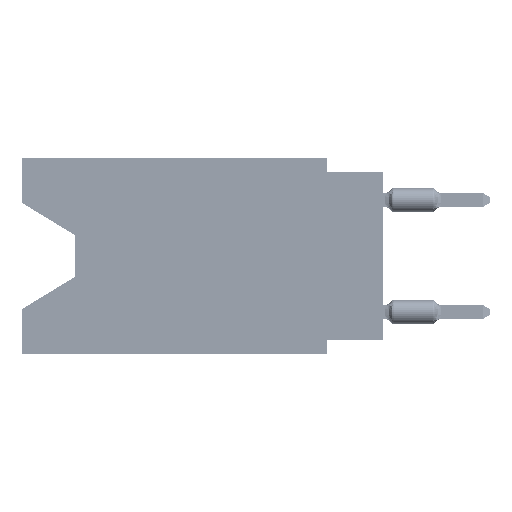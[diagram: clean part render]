
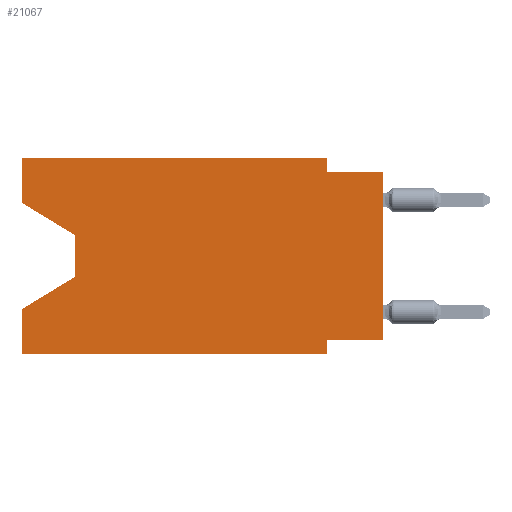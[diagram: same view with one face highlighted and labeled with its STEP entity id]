
A CAD part, left-side view. The second image highlights one B-rep face of the part: STEP entity #21067.
In plain terms, the highlighted planar face has unit normal (-1, 0, 0).
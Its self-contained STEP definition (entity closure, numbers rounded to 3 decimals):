
#1069 = DIRECTION ( 'NONE',  ( 0., -0.855, -0.519 ) ) ;
#2312 = EDGE_CURVE ( 'NONE', #9197, #61642, #28352, .T. ) ;
#5440 = DIRECTION ( 'NONE',  ( 0., 1., 0. ) ) ;
#7209 = LINE ( 'NONE', #52295, #49296 ) ;
#7264 = LINE ( 'NONE', #97376, #94020 ) ;
#8299 = VERTEX_POINT ( 'NONE', #86660 ) ;
#9197 = VERTEX_POINT ( 'NONE', #35222 ) ;
#9353 = EDGE_CURVE ( 'NONE', #62668, #56222, #99174, .T. ) ;
#10160 = VECTOR ( 'NONE', #47210, 1000. ) ;
#11792 = VECTOR ( 'NONE', #5440, 1000. ) ;
#11916 = EDGE_CURVE ( 'NONE', #56222, #8299, #92805, .T. ) ;
#14331 = CARTESIAN_POINT ( 'NONE',  ( 0., 0., -8.255 ) ) ;
#15845 = VECTOR ( 'NONE', #57086, 1000. ) ;
#16177 = DIRECTION ( 'NONE',  ( 0., 0., 1. ) ) ;
#17160 = VECTOR ( 'NONE', #99667, 1000. ) ;
#17402 = LINE ( 'NONE', #63619, #22855 ) ;
#17681 = ORIENTED_EDGE ( 'NONE', *, *, #2312, .F. ) ;
#17985 = CARTESIAN_POINT ( 'NONE',  ( 0., 13.97, -3.505 ) ) ;
#19372 = ORIENTED_EDGE ( 'NONE', *, *, #9353, .F. ) ;
#20920 = LINE ( 'NONE', #110980, #15845 ) ;
#21067 = ADVANCED_FACE ( 'NONE', ( #76289 ), #112415, .F. ) ;
#21550 = VECTOR ( 'NONE', #55060, 1000. ) ;
#22855 = VECTOR ( 'NONE', #36965, 1000. ) ;
#23311 = EDGE_CURVE ( 'NONE', #47791, #34414, #20920, .T. ) ;
#26901 = EDGE_CURVE ( 'NONE', #94471, #62668, #17402, .T. ) ;
#27769 = DIRECTION ( 'NONE',  ( 0., 0., -1. ) ) ;
#28352 = LINE ( 'NONE', #108926, #107234 ) ;
#28545 = EDGE_CURVE ( 'NONE', #50113, #61642, #7209, .T. ) ;
#32169 = LINE ( 'NONE', #14331, #11792 ) ;
#33930 = ORIENTED_EDGE ( 'NONE', *, *, #49506, .T. ) ;
#34414 = VERTEX_POINT ( 'NONE', #98135 ) ;
#35222 = CARTESIAN_POINT ( 'NONE',  ( 0., 2.54, -8.255 ) ) ;
#35524 = CARTESIAN_POINT ( 'NONE',  ( 0., 16.383, 0. ) ) ;
#36965 = DIRECTION ( 'NONE',  ( 0., -1., 0. ) ) ;
#38448 = VECTOR ( 'NONE', #73709, 1000. ) ;
#38910 = CARTESIAN_POINT ( 'NONE',  ( 0., 0., -0.635 ) ) ;
#40034 = VERTEX_POINT ( 'NONE', #108774 ) ;
#40104 = CARTESIAN_POINT ( 'NONE',  ( 0., 2.54, -8.89 ) ) ;
#45373 = CARTESIAN_POINT ( 'NONE',  ( 0., 16.383, 0. ) ) ;
#47210 = DIRECTION ( 'NONE',  ( 0., -1., 0. ) ) ;
#47679 = VERTEX_POINT ( 'NONE', #94489 ) ;
#47791 = VERTEX_POINT ( 'NONE', #17985 ) ;
#47864 = CARTESIAN_POINT ( 'NONE',  ( 0., 16.383, 0. ) ) ;
#49296 = VECTOR ( 'NONE', #88410, 1000. ) ;
#49506 = EDGE_CURVE ( 'NONE', #40034, #47791, #82264, .T. ) ;
#50113 = VERTEX_POINT ( 'NONE', #70050 ) ;
#52295 = CARTESIAN_POINT ( 'NONE',  ( 0., 16.383, -8.89 ) ) ;
#54598 = VERTEX_POINT ( 'NONE', #93763 ) ;
#55060 = DIRECTION ( 'NONE',  ( 0., 0., 1. ) ) ;
#56222 = VERTEX_POINT ( 'NONE', #82944 ) ;
#56693 = ORIENTED_EDGE ( 'NONE', *, *, #11916, .F. ) ;
#56772 = VECTOR ( 'NONE', #1069, 1000. ) ;
#57086 = DIRECTION ( 'NONE',  ( 0., 0., -1. ) ) ;
#57155 = AXIS2_PLACEMENT_3D ( 'NONE', #47864, #86310, #104099 ) ;
#57441 = LINE ( 'NONE', #103031, #89751 ) ;
#57734 = EDGE_CURVE ( 'NONE', #50113, #47679, #7264, .T. ) ;
#60188 = ORIENTED_EDGE ( 'NONE', *, *, #108642, .T. ) ;
#61642 = VERTEX_POINT ( 'NONE', #40104 ) ;
#62668 = VERTEX_POINT ( 'NONE', #64598 ) ;
#63619 = CARTESIAN_POINT ( 'NONE',  ( 0., 16.383, 0. ) ) ;
#64598 = CARTESIAN_POINT ( 'NONE',  ( 0., 2.54, 0. ) ) ;
#67486 = DIRECTION ( 'NONE',  ( 0., 0., 1. ) ) ;
#68733 = EDGE_LOOP ( 'NONE', ( #33930, #86900, #96023, #110494, #102686, #17681, #106634, #60188, #56693, #19372, #114359, #69051 ) ) ;
#69051 = ORIENTED_EDGE ( 'NONE', *, *, #92072, .F. ) ;
#70050 = CARTESIAN_POINT ( 'NONE',  ( 0., 16.383, -8.89 ) ) ;
#71059 = EDGE_CURVE ( 'NONE', #34414, #47679, #91371, .T. ) ;
#73263 = EDGE_CURVE ( 'NONE', #54598, #9197, #32169, .T. ) ;
#73709 = DIRECTION ( 'NONE',  ( 0., 0., -1. ) ) ;
#76289 = FACE_OUTER_BOUND ( 'NONE', #68733, .T. ) ;
#80528 = LINE ( 'NONE', #35524, #21550 ) ;
#81076 = CARTESIAN_POINT ( 'NONE',  ( 0., 16.383, -2.038 ) ) ;
#82264 = LINE ( 'NONE', #81076, #56772 ) ;
#82944 = CARTESIAN_POINT ( 'NONE',  ( 0., 2.54, -0.635 ) ) ;
#86310 = DIRECTION ( 'NONE',  ( 1., 0., 0. ) ) ;
#86660 = CARTESIAN_POINT ( 'NONE',  ( 0., 0., -0.635 ) ) ;
#86900 = ORIENTED_EDGE ( 'NONE', *, *, #23311, .T. ) ;
#88410 = DIRECTION ( 'NONE',  ( 0., -1., 0. ) ) ;
#89751 = VECTOR ( 'NONE', #67486, 1000. ) ;
#90860 = CARTESIAN_POINT ( 'NONE',  ( 0., 2.54, 0. ) ) ;
#91371 = LINE ( 'NONE', #107384, #17160 ) ;
#92072 = EDGE_CURVE ( 'NONE', #40034, #94471, #80528, .T. ) ;
#92805 = LINE ( 'NONE', #38910, #10160 ) ;
#93763 = CARTESIAN_POINT ( 'NONE',  ( 0., 0., -8.255 ) ) ;
#94020 = VECTOR ( 'NONE', #16177, 1000. ) ;
#94471 = VERTEX_POINT ( 'NONE', #45373 ) ;
#94489 = CARTESIAN_POINT ( 'NONE',  ( 0., 16.383, -6.852 ) ) ;
#96023 = ORIENTED_EDGE ( 'NONE', *, *, #71059, .T. ) ;
#97376 = CARTESIAN_POINT ( 'NONE',  ( 0., 16.383, 0. ) ) ;
#98135 = CARTESIAN_POINT ( 'NONE',  ( 0., 13.97, -5.385 ) ) ;
#99174 = LINE ( 'NONE', #90860, #38448 ) ;
#99667 = DIRECTION ( 'NONE',  ( 0., 0.855, -0.519 ) ) ;
#102686 = ORIENTED_EDGE ( 'NONE', *, *, #28545, .T. ) ;
#103031 = CARTESIAN_POINT ( 'NONE',  ( 0., 0., 0. ) ) ;
#104099 = DIRECTION ( 'NONE',  ( 0., 0., -1. ) ) ;
#106634 = ORIENTED_EDGE ( 'NONE', *, *, #73263, .F. ) ;
#107234 = VECTOR ( 'NONE', #27769, 1000. ) ;
#107384 = CARTESIAN_POINT ( 'NONE',  ( 0., 13.97, -5.385 ) ) ;
#108642 = EDGE_CURVE ( 'NONE', #54598, #8299, #57441, .T. ) ;
#108774 = CARTESIAN_POINT ( 'NONE',  ( 0., 16.383, -2.038 ) ) ;
#108926 = CARTESIAN_POINT ( 'NONE',  ( 0., 2.54, -8.89 ) ) ;
#110494 = ORIENTED_EDGE ( 'NONE', *, *, #57734, .F. ) ;
#110980 = CARTESIAN_POINT ( 'NONE',  ( 0., 13.97, -3.505 ) ) ;
#112415 = PLANE ( 'NONE',  #57155 ) ;
#114359 = ORIENTED_EDGE ( 'NONE', *, *, #26901, .F. ) ;
